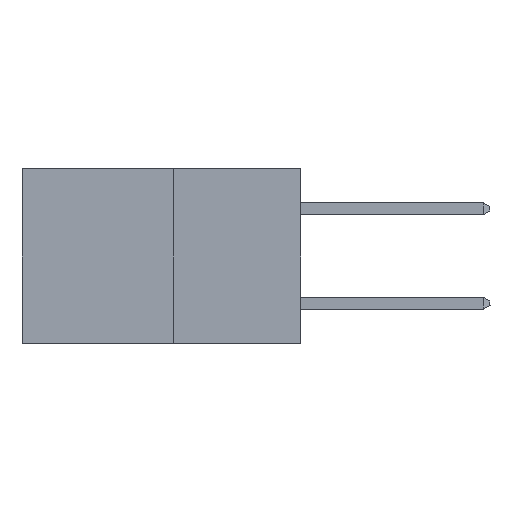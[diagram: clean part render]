
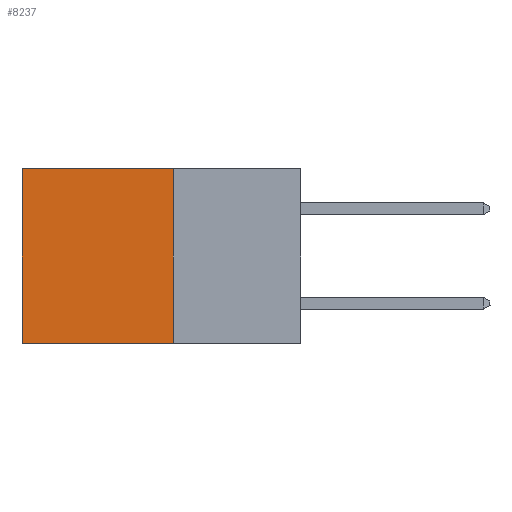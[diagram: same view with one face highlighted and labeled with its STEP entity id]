
A CAD part, left-side view. The second image highlights one B-rep face of the part: STEP entity #8237.
In plain terms, the highlighted planar face has unit normal (-1, 0, 0).
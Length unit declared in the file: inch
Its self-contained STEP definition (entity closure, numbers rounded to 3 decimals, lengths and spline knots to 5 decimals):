
#1094 = CARTESIAN_POINT ( 'NONE',  ( 0.277, 0.27, 0. ) ) ;
#3579 = LINE ( 'NONE', #13527, #8627 ) ;
#4302 = DIRECTION ( 'NONE',  ( 0., 1., 0. ) ) ;
#4408 = ORIENTED_EDGE ( 'NONE', *, *, #5948, .T. ) ;
#4601 = EDGE_CURVE ( 'NONE', #6143, #6406, #23685, .T. ) ;
#5948 = EDGE_CURVE ( 'NONE', #6143, #14173, #21875, .T. ) ;
#6120 = FACE_OUTER_BOUND ( 'NONE', #6847, .T. ) ;
#6131 = CARTESIAN_POINT ( 'NONE',  ( 0.277, 0.59, 0. ) ) ;
#6135 = VERTEX_POINT ( 'NONE', #10518 ) ;
#6143 = VERTEX_POINT ( 'NONE', #1094 ) ;
#6242 = AXIS2_PLACEMENT_3D ( 'NONE', #14142, #8530, #21712 ) ;
#6406 = VERTEX_POINT ( 'NONE', #9346 ) ;
#6847 = EDGE_LOOP ( 'NONE', ( #9090, #22914, #14704, #4408 ) ) ;
#8055 = DIRECTION ( 'NONE',  ( 0., 0., -1. ) ) ;
#8099 = VECTOR ( 'NONE', #8055, 39.37008 ) ;
#8237 = ADVANCED_FACE ( 'NONE', ( #6120 ), #17970, .F. ) ;
#8530 = DIRECTION ( 'NONE',  ( 1., 0., 0. ) ) ;
#8627 = VECTOR ( 'NONE', #9724, 39.37008 ) ;
#9090 = ORIENTED_EDGE ( 'NONE', *, *, #20899, .T. ) ;
#9346 = CARTESIAN_POINT ( 'NONE',  ( 0.277, 0.27, -0.37 ) ) ;
#9724 = DIRECTION ( 'NONE',  ( 0., 1., 0. ) ) ;
#9947 = CARTESIAN_POINT ( 'NONE',  ( 0.277, 0.27, 0. ) ) ;
#10518 = CARTESIAN_POINT ( 'NONE',  ( 0.277, 0.59, -0.37 ) ) ;
#11495 = CARTESIAN_POINT ( 'NONE',  ( 0.277, 0.27, -0.37 ) ) ;
#11568 = DIRECTION ( 'NONE',  ( 0., 0., -1. ) ) ;
#11880 = VECTOR ( 'NONE', #4302, 39.37008 ) ;
#12216 = VECTOR ( 'NONE', #11568, 39.37008 ) ;
#13527 = CARTESIAN_POINT ( 'NONE',  ( 0.277, 0.27, -0.37 ) ) ;
#14142 = CARTESIAN_POINT ( 'NONE',  ( 0.277, 0.27, -0.37 ) ) ;
#14173 = VERTEX_POINT ( 'NONE', #6131 ) ;
#14704 = ORIENTED_EDGE ( 'NONE', *, *, #4601, .F. ) ;
#17970 = PLANE ( 'NONE',  #6242 ) ;
#20899 = EDGE_CURVE ( 'NONE', #14173, #6135, #22201, .T. ) ;
#21529 = EDGE_CURVE ( 'NONE', #6406, #6135, #3579, .T. ) ;
#21712 = DIRECTION ( 'NONE',  ( 0., 0., -1. ) ) ;
#21875 = LINE ( 'NONE', #9947, #11880 ) ;
#22201 = LINE ( 'NONE', #22800, #12216 ) ;
#22800 = CARTESIAN_POINT ( 'NONE',  ( 0.277, 0.59, -0.37 ) ) ;
#22914 = ORIENTED_EDGE ( 'NONE', *, *, #21529, .F. ) ;
#23685 = LINE ( 'NONE', #11495, #8099 ) ;
